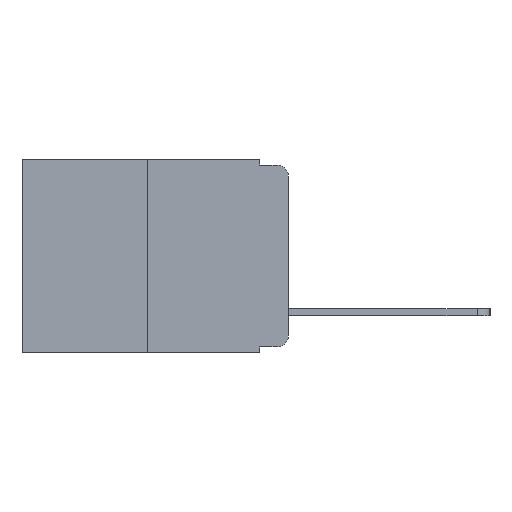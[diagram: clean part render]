
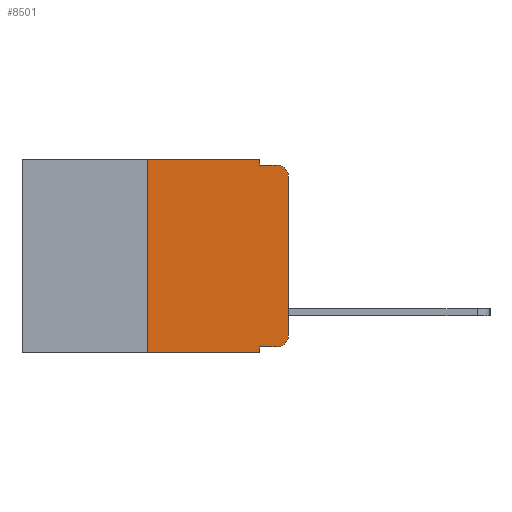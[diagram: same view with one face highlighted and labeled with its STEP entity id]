
A CAD part, left-side view. The second image highlights one B-rep face of the part: STEP entity #8501.
In plain terms, the highlighted planar face has unit normal (-1, 0, 0).
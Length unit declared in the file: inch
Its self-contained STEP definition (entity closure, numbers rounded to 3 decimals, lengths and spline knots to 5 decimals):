
#10 = ORIENTED_EDGE ( 'NONE', *, *, #1344, .F. ) ;
#111 = ORIENTED_EDGE ( 'NONE', *, *, #3755, .T. ) ;
#392 = CARTESIAN_POINT ( 'NONE',  ( 0., 0.051, 0. ) ) ;
#478 = DIRECTION ( 'NONE',  ( 0., 0., -1. ) ) ;
#511 = EDGE_CURVE ( 'NONE', #1196, #1006, #6174, .T. ) ;
#665 = ORIENTED_EDGE ( 'NONE', *, *, #12592, .T. ) ;
#728 = DIRECTION ( 'NONE',  ( 0., -1., 0. ) ) ;
#995 = VERTEX_POINT ( 'NONE', #4635 ) ;
#1006 = VERTEX_POINT ( 'NONE', #13641 ) ;
#1196 = VERTEX_POINT ( 'NONE', #10376 ) ;
#1344 = EDGE_CURVE ( 'NONE', #12033, #9532, #14276, .T. ) ;
#1709 = CARTESIAN_POINT ( 'NONE',  ( 0., 0.02, -0.313 ) ) ;
#1873 = VECTOR ( 'NONE', #478, 39.37008 ) ;
#1963 = CARTESIAN_POINT ( 'NONE',  ( 0., 0.051, -0.343 ) ) ;
#2157 = EDGE_CURVE ( 'NONE', #9532, #995, #12310, .T. ) ;
#2216 = CARTESIAN_POINT ( 'NONE',  ( 0., 0., -0.03 ) ) ;
#2430 = AXIS2_PLACEMENT_3D ( 'NONE', #1709, #9952, #2882 ) ;
#2843 = EDGE_CURVE ( 'NONE', #1006, #12033, #6522, .T. ) ;
#2865 = DIRECTION ( 'NONE',  ( 0., -1., 0. ) ) ;
#2882 = DIRECTION ( 'NONE',  ( 0., 0., -1. ) ) ;
#2893 = DIRECTION ( 'NONE',  ( 0., 0., -1. ) ) ;
#3166 = VERTEX_POINT ( 'NONE', #9193 ) ;
#3197 = VERTEX_POINT ( 'NONE', #1963 ) ;
#3284 = VECTOR ( 'NONE', #7943, 39.37008 ) ;
#3309 = DIRECTION ( 'NONE',  ( 1., 0., 0. ) ) ;
#3755 = EDGE_CURVE ( 'NONE', #5806, #995, #12792, .T. ) ;
#4556 = EDGE_CURVE ( 'NONE', #3166, #5806, #5403, .T. ) ;
#4635 = CARTESIAN_POINT ( 'NONE',  ( 0., 0.02, -0.01 ) ) ;
#4797 = AXIS2_PLACEMENT_3D ( 'NONE', #14169, #14149, #14130 ) ;
#4811 = DIRECTION ( 'NONE',  ( 0., 0., 1. ) ) ;
#4916 = CARTESIAN_POINT ( 'NONE',  ( 0., 0.051, -0.01 ) ) ;
#5157 = CARTESIAN_POINT ( 'NONE',  ( 0., 0., 0. ) ) ;
#5403 = LINE ( 'NONE', #5157, #11230 ) ;
#5806 = VERTEX_POINT ( 'NONE', #2216 ) ;
#5866 = EDGE_CURVE ( 'NONE', #1196, #3197, #9543, .T. ) ;
#6174 = LINE ( 'NONE', #7365, #8454 ) ;
#6194 = FACE_OUTER_BOUND ( 'NONE', #11090, .T. ) ;
#6293 = ORIENTED_EDGE ( 'NONE', *, *, #2157, .F. ) ;
#6522 = LINE ( 'NONE', #11542, #6886 ) ;
#6739 = VECTOR ( 'NONE', #2865, 39.37008 ) ;
#6886 = VECTOR ( 'NONE', #728, 39.37008 ) ;
#7365 = CARTESIAN_POINT ( 'NONE',  ( 0., 0.25, 0. ) ) ;
#7720 = ORIENTED_EDGE ( 'NONE', *, *, #5866, .T. ) ;
#7943 = DIRECTION ( 'NONE',  ( 0., -1., 0. ) ) ;
#7967 = PLANE ( 'NONE',  #10535 ) ;
#8088 = LINE ( 'NONE', #11132, #1873 ) ;
#8454 = VECTOR ( 'NONE', #4811, 39.37008 ) ;
#8501 = ADVANCED_FACE ( 'NONE', ( #6194 ), #7967, .F. ) ;
#8580 = CARTESIAN_POINT ( 'NONE',  ( 0., 0.051, 0. ) ) ;
#8649 = CARTESIAN_POINT ( 'NONE',  ( 0., 0.051, -0.333 ) ) ;
#8793 = ORIENTED_EDGE ( 'NONE', *, *, #13322, .T. ) ;
#8867 = VECTOR ( 'NONE', #14004, 39.37008 ) ;
#9193 = CARTESIAN_POINT ( 'NONE',  ( 0., 0., -0.313 ) ) ;
#9231 = VERTEX_POINT ( 'NONE', #10859 ) ;
#9532 = VERTEX_POINT ( 'NONE', #13021 ) ;
#9543 = LINE ( 'NONE', #12540, #3284 ) ;
#9849 = LINE ( 'NONE', #8649, #6739 ) ;
#9952 = DIRECTION ( 'NONE',  ( -1., 0., 0. ) ) ;
#10059 = CIRCLE ( 'NONE', #2430, 0.02 ) ;
#10376 = CARTESIAN_POINT ( 'NONE',  ( 0., 0.25, -0.343 ) ) ;
#10377 = CARTESIAN_POINT ( 'NONE',  ( 0., 0.473, 0. ) ) ;
#10535 = AXIS2_PLACEMENT_3D ( 'NONE', #10377, #3309, #11496 ) ;
#10774 = DIRECTION ( 'NONE',  ( 0., 0., 1. ) ) ;
#10859 = CARTESIAN_POINT ( 'NONE',  ( 0., 0.051, -0.333 ) ) ;
#10869 = VERTEX_POINT ( 'NONE', #14932 ) ;
#11090 = EDGE_LOOP ( 'NONE', ( #13140, #111, #6293, #10, #11707, #12303, #7720, #12241, #8793, #665 ) ) ;
#11132 = CARTESIAN_POINT ( 'NONE',  ( 0., 0.051, 0. ) ) ;
#11230 = VECTOR ( 'NONE', #10774, 39.37008 ) ;
#11394 = VECTOR ( 'NONE', #2893, 39.37008 ) ;
#11496 = DIRECTION ( 'NONE',  ( 0., 0., -1. ) ) ;
#11542 = CARTESIAN_POINT ( 'NONE',  ( 0., 0.473, 0. ) ) ;
#11707 = ORIENTED_EDGE ( 'NONE', *, *, #2843, .F. ) ;
#12033 = VERTEX_POINT ( 'NONE', #8580 ) ;
#12241 = ORIENTED_EDGE ( 'NONE', *, *, #14021, .F. ) ;
#12303 = ORIENTED_EDGE ( 'NONE', *, *, #511, .F. ) ;
#12310 = LINE ( 'NONE', #4916, #8867 ) ;
#12540 = CARTESIAN_POINT ( 'NONE',  ( 0., 0.473, -0.343 ) ) ;
#12592 = EDGE_CURVE ( 'NONE', #10869, #3166, #10059, .T. ) ;
#12792 = CIRCLE ( 'NONE', #4797, 0.02 ) ;
#13021 = CARTESIAN_POINT ( 'NONE',  ( 0., 0.051, -0.01 ) ) ;
#13140 = ORIENTED_EDGE ( 'NONE', *, *, #4556, .T. ) ;
#13322 = EDGE_CURVE ( 'NONE', #9231, #10869, #9849, .T. ) ;
#13641 = CARTESIAN_POINT ( 'NONE',  ( 0., 0.25, 0. ) ) ;
#14004 = DIRECTION ( 'NONE',  ( 0., -1., 0. ) ) ;
#14021 = EDGE_CURVE ( 'NONE', #9231, #3197, #8088, .T. ) ;
#14130 = DIRECTION ( 'NONE',  ( 0., 0., -1. ) ) ;
#14149 = DIRECTION ( 'NONE',  ( -1., 0., 0. ) ) ;
#14169 = CARTESIAN_POINT ( 'NONE',  ( 0., 0.02, -0.03 ) ) ;
#14276 = LINE ( 'NONE', #392, #11394 ) ;
#14932 = CARTESIAN_POINT ( 'NONE',  ( 0., 0.02, -0.333 ) ) ;
